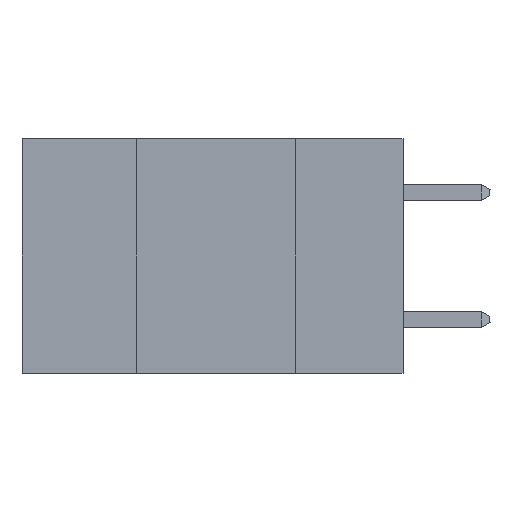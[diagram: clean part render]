
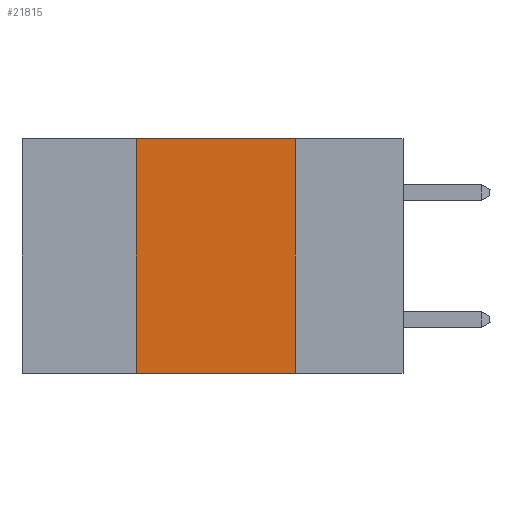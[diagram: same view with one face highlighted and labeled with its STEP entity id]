
A CAD part, left-side view. The second image highlights one B-rep face of the part: STEP entity #21815.
In plain terms, the highlighted planar face has unit normal (-1, 0, 0).
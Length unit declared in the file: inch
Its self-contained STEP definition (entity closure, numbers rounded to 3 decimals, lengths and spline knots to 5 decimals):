
#815 = CARTESIAN_POINT ( 'NONE',  ( 0., 0.42, 0. ) ) ;
#4750 = EDGE_CURVE ( 'NONE', #39255, #9377, #36578, .T. ) ;
#5106 = VERTEX_POINT ( 'NONE', #31116 ) ;
#5219 = CARTESIAN_POINT ( 'NONE',  ( 0., 0.6, -0.37 ) ) ;
#5439 = PLANE ( 'NONE',  #15808 ) ;
#7375 = CARTESIAN_POINT ( 'NONE',  ( 0., 0.42, 0. ) ) ;
#7743 = DIRECTION ( 'NONE',  ( 0., -1., 0. ) ) ;
#8070 = LINE ( 'NONE', #5219, #16097 ) ;
#8323 = EDGE_CURVE ( 'NONE', #9713, #39255, #28994, .T. ) ;
#9358 = FACE_OUTER_BOUND ( 'NONE', #36199, .T. ) ;
#9377 = VERTEX_POINT ( 'NONE', #9971 ) ;
#9713 = VERTEX_POINT ( 'NONE', #7375 ) ;
#9971 = CARTESIAN_POINT ( 'NONE',  ( 0., 0.17, -0.37 ) ) ;
#11960 = DIRECTION ( 'NONE',  ( 0., 0., -1. ) ) ;
#14978 = DIRECTION ( 'NONE',  ( 0., -1., 0. ) ) ;
#15021 = VECTOR ( 'NONE', #11960, 39.37008 ) ;
#15421 = EDGE_CURVE ( 'NONE', #5106, #9377, #8070, .T. ) ;
#15808 = AXIS2_PLACEMENT_3D ( 'NONE', #21690, #28101, #41241 ) ;
#16097 = VECTOR ( 'NONE', #14978, 39.37008 ) ;
#17907 = VECTOR ( 'NONE', #33040, 39.37008 ) ;
#18926 = ORIENTED_EDGE ( 'NONE', *, *, #15421, .T. ) ;
#20538 = VECTOR ( 'NONE', #7743, 39.37008 ) ;
#21690 = CARTESIAN_POINT ( 'NONE',  ( 0., 0.6, 0. ) ) ;
#21815 = ADVANCED_FACE ( 'NONE', ( #9358 ), #5439, .F. ) ;
#21932 = EDGE_CURVE ( 'NONE', #5106, #9713, #22843, .T. ) ;
#22194 = ORIENTED_EDGE ( 'NONE', *, *, #4750, .F. ) ;
#22843 = LINE ( 'NONE', #815, #17907 ) ;
#23911 = CARTESIAN_POINT ( 'NONE',  ( 0., 0.17, 0. ) ) ;
#27813 = ORIENTED_EDGE ( 'NONE', *, *, #21932, .F. ) ;
#28101 = DIRECTION ( 'NONE',  ( 1., 0., 0. ) ) ;
#28994 = LINE ( 'NONE', #30562, #20538 ) ;
#30562 = CARTESIAN_POINT ( 'NONE',  ( 0., 0.6, 0. ) ) ;
#31116 = CARTESIAN_POINT ( 'NONE',  ( 0., 0.42, -0.37 ) ) ;
#31406 = ORIENTED_EDGE ( 'NONE', *, *, #8323, .F. ) ;
#33040 = DIRECTION ( 'NONE',  ( 0., 0., 1. ) ) ;
#36199 = EDGE_LOOP ( 'NONE', ( #22194, #31406, #27813, #18926 ) ) ;
#36578 = LINE ( 'NONE', #37301, #15021 ) ;
#37301 = CARTESIAN_POINT ( 'NONE',  ( 0., 0.17, 0. ) ) ;
#39255 = VERTEX_POINT ( 'NONE', #23911 ) ;
#41241 = DIRECTION ( 'NONE',  ( 0., 0., -1. ) ) ;
